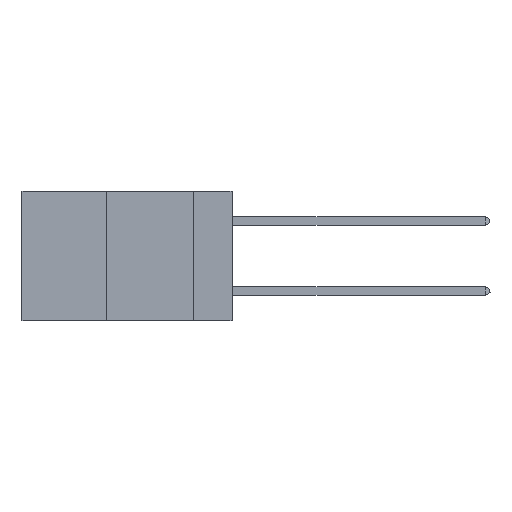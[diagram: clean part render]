
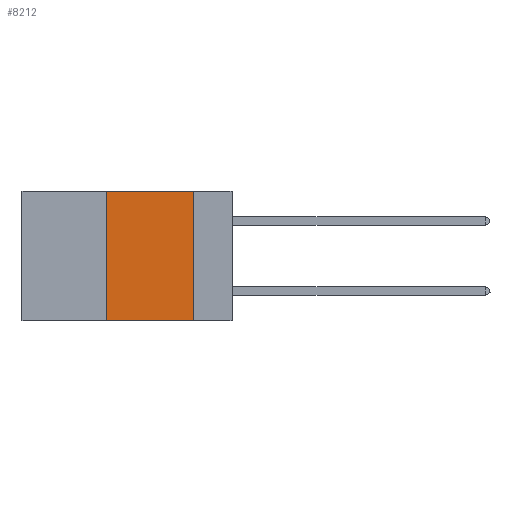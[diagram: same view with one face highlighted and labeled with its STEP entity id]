
A CAD part, left-side view. The second image highlights one B-rep face of the part: STEP entity #8212.
In plain terms, the highlighted planar face has unit normal (-1, 0, 0).
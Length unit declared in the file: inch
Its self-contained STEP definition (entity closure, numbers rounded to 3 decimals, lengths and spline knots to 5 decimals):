
#627 = EDGE_CURVE ( 'NONE', #1790, #10249, #12879, .T. ) ;
#712 = VECTOR ( 'NONE', #13158, 39.37008 ) ;
#1130 = CARTESIAN_POINT ( 'NONE',  ( 0., 0.36, 0. ) ) ;
#1367 = ORIENTED_EDGE ( 'NONE', *, *, #7415, .T. ) ;
#1472 = CARTESIAN_POINT ( 'NONE',  ( 0., 0.11, 0. ) ) ;
#1592 = VECTOR ( 'NONE', #2800, 39.37008 ) ;
#1790 = VERTEX_POINT ( 'NONE', #1472 ) ;
#2800 = DIRECTION ( 'NONE',  ( 0., -1., 0. ) ) ;
#3167 = DIRECTION ( 'NONE',  ( 1., 0., 0. ) ) ;
#3235 = VECTOR ( 'NONE', #5139, 39.37008 ) ;
#4015 = AXIS2_PLACEMENT_3D ( 'NONE', #4040, #3167, #12446 ) ;
#4040 = CARTESIAN_POINT ( 'NONE',  ( 0., 0.6, 0. ) ) ;
#4469 = CARTESIAN_POINT ( 'NONE',  ( 0., 0.36, 0. ) ) ;
#4921 = CARTESIAN_POINT ( 'NONE',  ( 0., 0.6, -0.37 ) ) ;
#5139 = DIRECTION ( 'NONE',  ( 0., -1., 0. ) ) ;
#5508 = DIRECTION ( 'NONE',  ( 0., 0., -1. ) ) ;
#5581 = ORIENTED_EDGE ( 'NONE', *, *, #627, .F. ) ;
#7415 = EDGE_CURVE ( 'NONE', #7861, #10249, #14316, .T. ) ;
#7861 = VERTEX_POINT ( 'NONE', #14496 ) ;
#8212 = ADVANCED_FACE ( 'NONE', ( #11153 ), #11310, .F. ) ;
#8914 = CARTESIAN_POINT ( 'NONE',  ( 0., 0.6, 0. ) ) ;
#10140 = ORIENTED_EDGE ( 'NONE', *, *, #15263, .F. ) ;
#10249 = VERTEX_POINT ( 'NONE', #11160 ) ;
#11083 = CARTESIAN_POINT ( 'NONE',  ( 0., 0.11, 0. ) ) ;
#11153 = FACE_OUTER_BOUND ( 'NONE', #15344, .T. ) ;
#11160 = CARTESIAN_POINT ( 'NONE',  ( 0., 0.11, -0.37 ) ) ;
#11310 = PLANE ( 'NONE',  #4015 ) ;
#12135 = EDGE_CURVE ( 'NONE', #14499, #1790, #12667, .T. ) ;
#12179 = LINE ( 'NONE', #4469, #712 ) ;
#12446 = DIRECTION ( 'NONE',  ( 0., 0., -1. ) ) ;
#12667 = LINE ( 'NONE', #8914, #1592 ) ;
#12879 = LINE ( 'NONE', #11083, #14049 ) ;
#13158 = DIRECTION ( 'NONE',  ( 0., 0., 1. ) ) ;
#14049 = VECTOR ( 'NONE', #5508, 39.37008 ) ;
#14316 = LINE ( 'NONE', #4921, #3235 ) ;
#14496 = CARTESIAN_POINT ( 'NONE',  ( 0., 0.36, -0.37 ) ) ;
#14499 = VERTEX_POINT ( 'NONE', #1130 ) ;
#15263 = EDGE_CURVE ( 'NONE', #7861, #14499, #12179, .T. ) ;
#15344 = EDGE_LOOP ( 'NONE', ( #5581, #16089, #10140, #1367 ) ) ;
#16089 = ORIENTED_EDGE ( 'NONE', *, *, #12135, .F. ) ;
